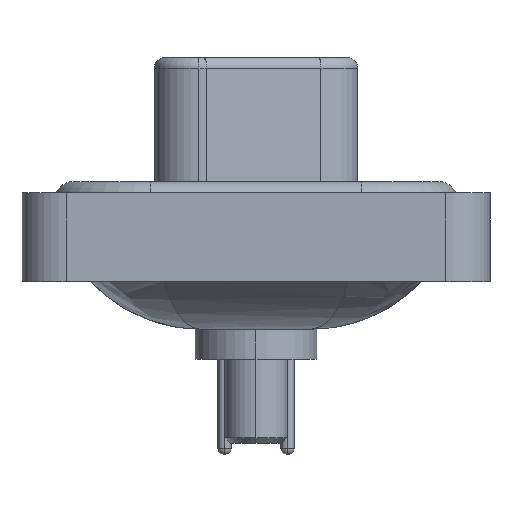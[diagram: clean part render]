
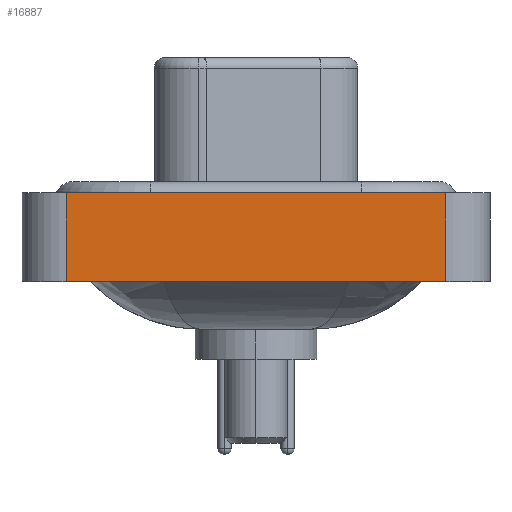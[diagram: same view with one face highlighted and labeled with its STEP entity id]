
A CAD part, left-side view. The second image highlights one B-rep face of the part: STEP entity #16887.
In plain terms, the highlighted planar face has unit normal (-1, 0, 0).
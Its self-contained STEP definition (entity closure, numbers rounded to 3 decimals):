
#601 = CARTESIAN_POINT ( 'NONE',  ( -7.35, 8.55, 0.4 ) ) ;
#1049 = VECTOR ( 'NONE', #6057, 1000. ) ;
#1067 = CARTESIAN_POINT ( 'NONE',  ( -7.35, -8.55, -3.6 ) ) ;
#2113 = AXIS2_PLACEMENT_3D ( 'NONE', #16423, #19861, #4745 ) ;
#2247 = LINE ( 'NONE', #7207, #5964 ) ;
#4009 = DIRECTION ( 'NONE',  ( 0., 0., 1. ) ) ;
#4116 = DIRECTION ( 'NONE',  ( 0., -1., 0. ) ) ;
#4216 = CARTESIAN_POINT ( 'NONE',  ( -7.35, -8.55, 0.4 ) ) ;
#4279 = EDGE_CURVE ( 'NONE', #12451, #7612, #17588, .T. ) ;
#4370 = ORIENTED_EDGE ( 'NONE', *, *, #12864, .F. ) ;
#4745 = DIRECTION ( 'NONE',  ( 0., 0., 1. ) ) ;
#5830 = LINE ( 'NONE', #14641, #1049 ) ;
#5964 = VECTOR ( 'NONE', #4009, 1000. ) ;
#6057 = DIRECTION ( 'NONE',  ( 0., -1., 0. ) ) ;
#7207 = CARTESIAN_POINT ( 'NONE',  ( -7.35, -8.55, -3.6 ) ) ;
#7612 = VERTEX_POINT ( 'NONE', #1067 ) ;
#7909 = EDGE_CURVE ( 'NONE', #7612, #19048, #2247, .T. ) ;
#9213 = ORIENTED_EDGE ( 'NONE', *, *, #13333, .F. ) ;
#9276 = PLANE ( 'NONE',  #2113 ) ;
#9895 = ORIENTED_EDGE ( 'NONE', *, *, #7909, .T. ) ;
#10061 = VERTEX_POINT ( 'NONE', #601 ) ;
#10189 = VECTOR ( 'NONE', #14164, 1000. ) ;
#10738 = CARTESIAN_POINT ( 'NONE',  ( -7.35, -8.55, -3.6 ) ) ;
#10748 = ORIENTED_EDGE ( 'NONE', *, *, #4279, .T. ) ;
#12451 = VERTEX_POINT ( 'NONE', #20599 ) ;
#12727 = CARTESIAN_POINT ( 'NONE',  ( -7.35, 8.55, -3.6 ) ) ;
#12864 = EDGE_CURVE ( 'NONE', #12451, #10061, #21116, .T. ) ;
#13127 = FACE_OUTER_BOUND ( 'NONE', #17411, .T. ) ;
#13333 = EDGE_CURVE ( 'NONE', #10061, #19048, #5830, .T. ) ;
#14164 = DIRECTION ( 'NONE',  ( 0., 0., 1. ) ) ;
#14641 = CARTESIAN_POINT ( 'NONE',  ( -7.35, -8.55, 0.4 ) ) ;
#16423 = CARTESIAN_POINT ( 'NONE',  ( -7.35, -8.55, -3.6 ) ) ;
#16887 = ADVANCED_FACE ( 'NONE', ( #13127 ), #9276, .T. ) ;
#17411 = EDGE_LOOP ( 'NONE', ( #9895, #9213, #4370, #10748 ) ) ;
#17588 = LINE ( 'NONE', #10738, #17833 ) ;
#17833 = VECTOR ( 'NONE', #4116, 1000. ) ;
#19048 = VERTEX_POINT ( 'NONE', #4216 ) ;
#19861 = DIRECTION ( 'NONE',  ( -1., 0., 0. ) ) ;
#20599 = CARTESIAN_POINT ( 'NONE',  ( -7.35, 8.55, -3.6 ) ) ;
#21116 = LINE ( 'NONE', #12727, #10189 ) ;
